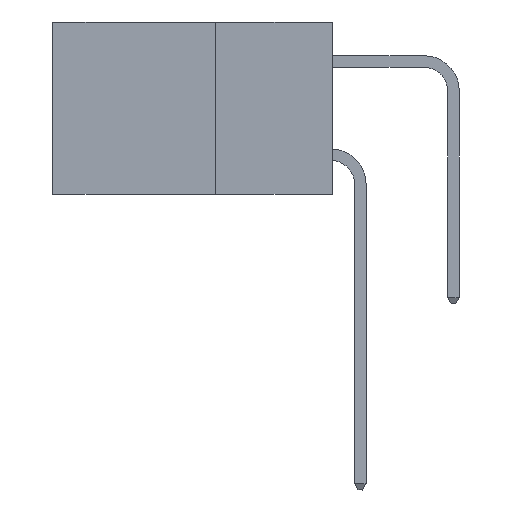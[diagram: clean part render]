
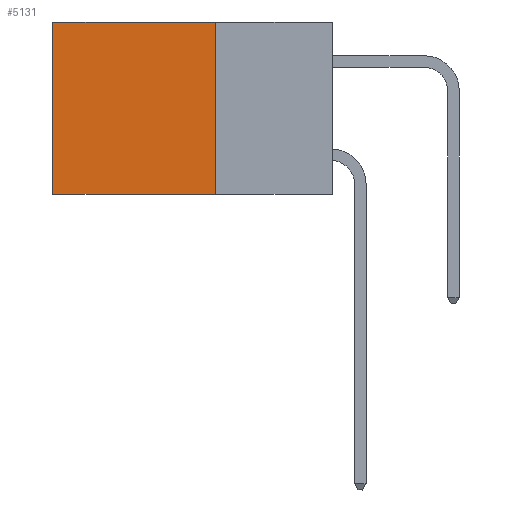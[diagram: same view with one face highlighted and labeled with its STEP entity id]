
A CAD part, left-side view. The second image highlights one B-rep face of the part: STEP entity #5131.
In plain terms, the highlighted planar face has unit normal (-1, 0, 0).
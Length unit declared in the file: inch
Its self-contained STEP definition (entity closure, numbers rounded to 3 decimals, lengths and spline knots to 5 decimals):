
#88 = CARTESIAN_POINT ( 'NONE',  ( 0.2615, 0.25, 0. ) ) ;
#299 = EDGE_CURVE ( 'NONE', #3077, #7120, #1826, .T. ) ;
#606 = VERTEX_POINT ( 'NONE', #9176 ) ;
#727 = EDGE_CURVE ( 'NONE', #606, #8172, #10176, .T. ) ;
#792 = DIRECTION ( 'NONE',  ( 0., 0., -1. ) ) ;
#938 = AXIS2_PLACEMENT_3D ( 'NONE', #2865, #8361, #8568 ) ;
#1187 = DIRECTION ( 'NONE',  ( 0., 0., -1. ) ) ;
#1402 = PLANE ( 'NONE',  #938 ) ;
#1447 = VECTOR ( 'NONE', #1187, 39.37008 ) ;
#1472 = EDGE_CURVE ( 'NONE', #3077, #606, #4883, .T. ) ;
#1588 = VECTOR ( 'NONE', #1798, 39.37008 ) ;
#1798 = DIRECTION ( 'NONE',  ( 0., 1., 0. ) ) ;
#1826 = LINE ( 'NONE', #88, #8097 ) ;
#2153 = EDGE_CURVE ( 'NONE', #7120, #8172, #3515, .T. ) ;
#2279 = EDGE_LOOP ( 'NONE', ( #2543, #9486, #3403, #5039 ) ) ;
#2543 = ORIENTED_EDGE ( 'NONE', *, *, #2153, .T. ) ;
#2582 = CARTESIAN_POINT ( 'NONE',  ( 0.2615, 0.25, -0.37 ) ) ;
#2865 = CARTESIAN_POINT ( 'NONE',  ( 0.2615, 0.25, -0.37 ) ) ;
#3077 = VERTEX_POINT ( 'NONE', #6427 ) ;
#3403 = ORIENTED_EDGE ( 'NONE', *, *, #1472, .F. ) ;
#3515 = LINE ( 'NONE', #6723, #1447 ) ;
#4883 = LINE ( 'NONE', #2582, #9933 ) ;
#5039 = ORIENTED_EDGE ( 'NONE', *, *, #299, .T. ) ;
#5131 = ADVANCED_FACE ( 'NONE', ( #6770 ), #1402, .F. ) ;
#5628 = DIRECTION ( 'NONE',  ( 0., 1., 0. ) ) ;
#6331 = CARTESIAN_POINT ( 'NONE',  ( 0.2615, 0.6, 0. ) ) ;
#6427 = CARTESIAN_POINT ( 'NONE',  ( 0.2615, 0.25, 0. ) ) ;
#6723 = CARTESIAN_POINT ( 'NONE',  ( 0.2615, 0.6, -0.37 ) ) ;
#6770 = FACE_OUTER_BOUND ( 'NONE', #2279, .T. ) ;
#7120 = VERTEX_POINT ( 'NONE', #6331 ) ;
#8097 = VECTOR ( 'NONE', #5628, 39.37008 ) ;
#8172 = VERTEX_POINT ( 'NONE', #8889 ) ;
#8361 = DIRECTION ( 'NONE',  ( 1., 0., 0. ) ) ;
#8568 = DIRECTION ( 'NONE',  ( 0., 0., -1. ) ) ;
#8889 = CARTESIAN_POINT ( 'NONE',  ( 0.2615, 0.6, -0.37 ) ) ;
#9176 = CARTESIAN_POINT ( 'NONE',  ( 0.2615, 0.25, -0.37 ) ) ;
#9395 = CARTESIAN_POINT ( 'NONE',  ( 0.2615, 0.25, -0.37 ) ) ;
#9486 = ORIENTED_EDGE ( 'NONE', *, *, #727, .F. ) ;
#9933 = VECTOR ( 'NONE', #792, 39.37008 ) ;
#10176 = LINE ( 'NONE', #9395, #1588 ) ;
